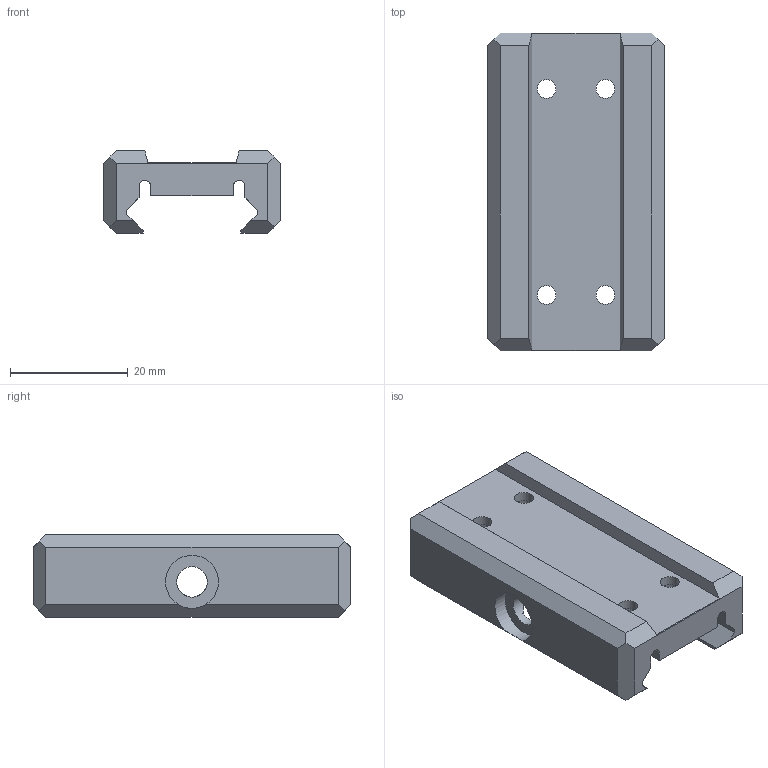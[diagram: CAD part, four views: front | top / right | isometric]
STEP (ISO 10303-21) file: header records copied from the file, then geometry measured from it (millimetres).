
FILE_DESCRIPTION(('FreeCAD Model'),'2;1');
FILE_NAME('Open CASCADE Shape Model','2025-08-02T21:24:37',(''),(''), 'Open CASCADE STEP processor 7.8','FreeCAD','Unknown');
FILE_SCHEMA(('AUTOMOTIVE_DESIGN { 1 0 10303 214 1 1 1 1 }'));
Length unit declared in the file: millimetre
Products named in the file (1): difference001
Bounding box: 30 x 54 x 14 mm (x, y, z)
Volume: 12023.2 mm3; surface area: 6806.3 mm2
Topology: 1 solids, 1 shells, 79 faces, 237 edges, 158 vertices
Faces by surface type: plane 65, cylinder 14
Full cylindrical faces by diameter (mm): 3.2 x4, 5.2 x2, 6 x4, 9 x1
Entity records: 3137 total; most frequent: CARTESIAN_POINT 931, ORIENTED_EDGE 474, DIRECTION 431, EDGE_CURVE 237, LINE 183, VECTOR 183, VERTEX_POINT 158, AXIS2_PLACEMENT_3D 124
